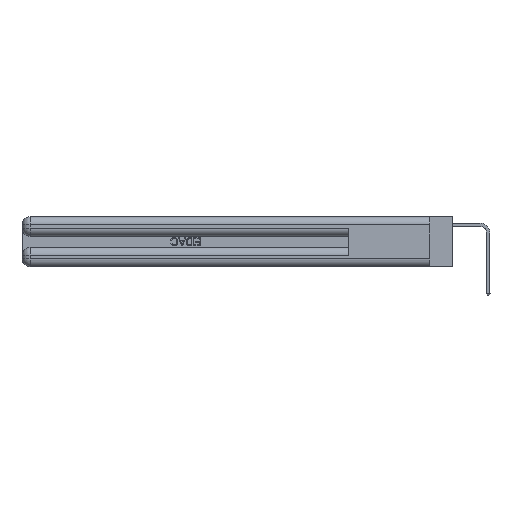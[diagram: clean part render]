
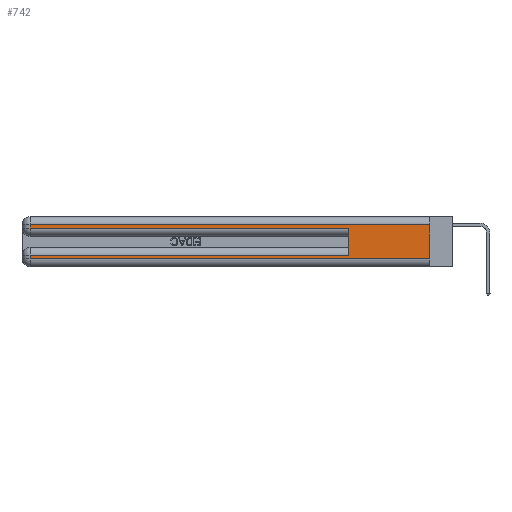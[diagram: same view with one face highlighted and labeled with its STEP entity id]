
A CAD part, left-side view. The second image highlights one B-rep face of the part: STEP entity #742.
In plain terms, the highlighted planar face has unit normal (-1, 0, 0).
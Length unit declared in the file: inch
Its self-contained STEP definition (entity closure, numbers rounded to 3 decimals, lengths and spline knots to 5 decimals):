
#742 = ADVANCED_FACE ( 'NONE', ( #3174 ), #30115, .F. ) ;
#1057 = VERTEX_POINT ( 'NONE', #2101 ) ;
#1182 = CARTESIAN_POINT ( 'NONE',  ( 0., 0.6, 0.085 ) ) ;
#1964 = AXIS2_PLACEMENT_3D ( 'NONE', #13764, #14281, #11168 ) ;
#2101 = CARTESIAN_POINT ( 'NONE',  ( 0., 2.94, 0.085 ) ) ;
#2214 = VECTOR ( 'NONE', #24483, 39.37008 ) ;
#2302 = CARTESIAN_POINT ( 'NONE',  ( 0., 2.94, 0.06 ) ) ;
#2383 = VECTOR ( 'NONE', #31038, 39.37008 ) ;
#2489 = CARTESIAN_POINT ( 'NONE',  ( 0., 0., 0.06 ) ) ;
#2948 = DIRECTION ( 'NONE',  ( 0., -1., 0. ) ) ;
#3174 = FACE_OUTER_BOUND ( 'NONE', #4827, .T. ) ;
#3431 = CARTESIAN_POINT ( 'NONE',  ( 0., 0., 0.31 ) ) ;
#4217 = VECTOR ( 'NONE', #2948, 39.37008 ) ;
#4441 = DIRECTION ( 'NONE',  ( 0., 1., 0. ) ) ;
#4827 = EDGE_LOOP ( 'NONE', ( #25321, #25871, #11941, #24983, #31316, #32380, #27157, #19818 ) ) ;
#6822 = EDGE_CURVE ( 'NONE', #9100, #9830, #8396, .T. ) ;
#7544 = LINE ( 'NONE', #31179, #14397 ) ;
#7748 = CARTESIAN_POINT ( 'NONE',  ( 0., 2.94, 0.37 ) ) ;
#8018 = DIRECTION ( 'NONE',  ( 0., 1., 0. ) ) ;
#8296 = LINE ( 'NONE', #13856, #2214 ) ;
#8396 = LINE ( 'NONE', #19015, #28821 ) ;
#9081 = EDGE_CURVE ( 'NONE', #33372, #16058, #8296, .T. ) ;
#9100 = VERTEX_POINT ( 'NONE', #3431 ) ;
#9830 = VERTEX_POINT ( 'NONE', #2489 ) ;
#11168 = DIRECTION ( 'NONE',  ( 0., 0., -1. ) ) ;
#11458 = LINE ( 'NONE', #32481, #4217 ) ;
#11941 = ORIENTED_EDGE ( 'NONE', *, *, #20099, .T. ) ;
#13711 = EDGE_CURVE ( 'NONE', #23450, #9830, #11458, .T. ) ;
#13762 = EDGE_CURVE ( 'NONE', #22088, #16058, #18606, .T. ) ;
#13764 = CARTESIAN_POINT ( 'NONE',  ( 0., 0., 0.37 ) ) ;
#13856 = CARTESIAN_POINT ( 'NONE',  ( 0., 0.6, 0.145 ) ) ;
#14281 = DIRECTION ( 'NONE',  ( 1., 0., 0. ) ) ;
#14397 = VECTOR ( 'NONE', #4441, 39.37008 ) ;
#15191 = DIRECTION ( 'NONE',  ( 0., 0., -1. ) ) ;
#16058 = VERTEX_POINT ( 'NONE', #23672 ) ;
#17956 = LINE ( 'NONE', #21261, #20195 ) ;
#18606 = LINE ( 'NONE', #29216, #21968 ) ;
#19015 = CARTESIAN_POINT ( 'NONE',  ( 0., 0., 0.37 ) ) ;
#19818 = ORIENTED_EDGE ( 'NONE', *, *, #13711, .T. ) ;
#20086 = EDGE_CURVE ( 'NONE', #9100, #24081, #7544, .T. ) ;
#20099 = EDGE_CURVE ( 'NONE', #24081, #22088, #33949, .T. ) ;
#20195 = VECTOR ( 'NONE', #8018, 39.37008 ) ;
#21261 = CARTESIAN_POINT ( 'NONE',  ( 0., 0., 0.085 ) ) ;
#21397 = DIRECTION ( 'NONE',  ( 0., -1., 0. ) ) ;
#21968 = VECTOR ( 'NONE', #21397, 39.37008 ) ;
#22088 = VERTEX_POINT ( 'NONE', #25226 ) ;
#22765 = VECTOR ( 'NONE', #15191, 39.37008 ) ;
#23235 = LINE ( 'NONE', #7748, #2383 ) ;
#23450 = VERTEX_POINT ( 'NONE', #2302 ) ;
#23672 = CARTESIAN_POINT ( 'NONE',  ( 0., 0.6, 0.285 ) ) ;
#24081 = VERTEX_POINT ( 'NONE', #32817 ) ;
#24483 = DIRECTION ( 'NONE',  ( 0., 0., 1. ) ) ;
#24983 = ORIENTED_EDGE ( 'NONE', *, *, #13762, .T. ) ;
#25226 = CARTESIAN_POINT ( 'NONE',  ( 0., 2.94, 0.285 ) ) ;
#25321 = ORIENTED_EDGE ( 'NONE', *, *, #6822, .F. ) ;
#25812 = CARTESIAN_POINT ( 'NONE',  ( 0., 2.94, 0.37 ) ) ;
#25871 = ORIENTED_EDGE ( 'NONE', *, *, #20086, .T. ) ;
#26068 = EDGE_CURVE ( 'NONE', #1057, #23450, #23235, .T. ) ;
#27007 = DIRECTION ( 'NONE',  ( 0., 0., -1. ) ) ;
#27157 = ORIENTED_EDGE ( 'NONE', *, *, #26068, .T. ) ;
#28305 = EDGE_CURVE ( 'NONE', #33372, #1057, #17956, .T. ) ;
#28821 = VECTOR ( 'NONE', #27007, 39.37008 ) ;
#29216 = CARTESIAN_POINT ( 'NONE',  ( 0., 0., 0.285 ) ) ;
#30115 = PLANE ( 'NONE',  #1964 ) ;
#31038 = DIRECTION ( 'NONE',  ( 0., 0., -1. ) ) ;
#31179 = CARTESIAN_POINT ( 'NONE',  ( 0., 0., 0.31 ) ) ;
#31316 = ORIENTED_EDGE ( 'NONE', *, *, #9081, .F. ) ;
#32380 = ORIENTED_EDGE ( 'NONE', *, *, #28305, .T. ) ;
#32481 = CARTESIAN_POINT ( 'NONE',  ( 0., 0., 0.06 ) ) ;
#32817 = CARTESIAN_POINT ( 'NONE',  ( 0., 2.94, 0.31 ) ) ;
#33372 = VERTEX_POINT ( 'NONE', #1182 ) ;
#33949 = LINE ( 'NONE', #25812, #22765 ) ;
